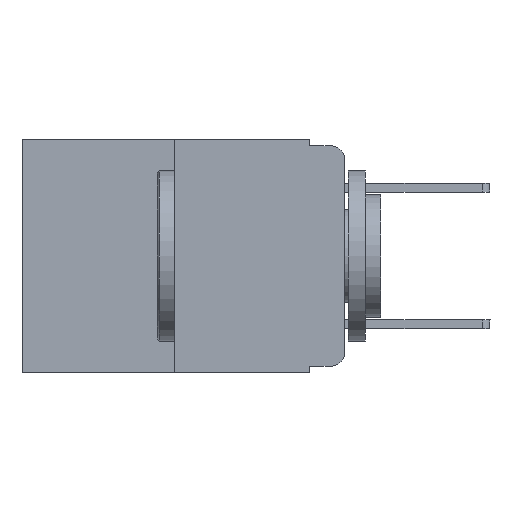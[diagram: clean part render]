
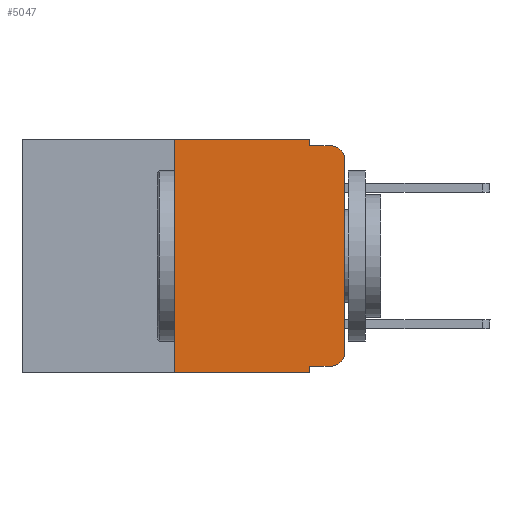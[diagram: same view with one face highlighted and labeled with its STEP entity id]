
A CAD part, left-side view. The second image highlights one B-rep face of the part: STEP entity #5047.
In plain terms, the highlighted planar face has unit normal (-1, 0, 0).
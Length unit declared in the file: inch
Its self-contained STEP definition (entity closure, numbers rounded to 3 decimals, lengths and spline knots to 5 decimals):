
#68 = EDGE_CURVE ( 'NONE', #5482, #10175, #2040, .T. ) ;
#242 = VECTOR ( 'NONE', #7209, 39.37008 ) ;
#312 = DIRECTION ( 'NONE',  ( 0., 0., -1. ) ) ;
#369 = LINE ( 'NONE', #2445, #910 ) ;
#607 = VERTEX_POINT ( 'NONE', #10407 ) ;
#863 = LINE ( 'NONE', #7872, #934 ) ;
#910 = VECTOR ( 'NONE', #6473, 39.37008 ) ;
#934 = VECTOR ( 'NONE', #11919, 39.37008 ) ;
#961 = CARTESIAN_POINT ( 'NONE',  ( 0., 0.25, -0.343 ) ) ;
#1066 = AXIS2_PLACEMENT_3D ( 'NONE', #4052, #8057, #12096 ) ;
#1186 = EDGE_CURVE ( 'NONE', #3997, #4994, #5885, .T. ) ;
#1191 = CARTESIAN_POINT ( 'NONE',  ( 0., 0.25, 0. ) ) ;
#1307 = LINE ( 'NONE', #9463, #3314 ) ;
#1376 = ORIENTED_EDGE ( 'NONE', *, *, #6485, .F. ) ;
#1532 = CIRCLE ( 'NONE', #11672, 0.02 ) ;
#1916 = CARTESIAN_POINT ( 'NONE',  ( 0., 0.051, -0.01 ) ) ;
#1965 = EDGE_CURVE ( 'NONE', #12081, #3352, #12812, .T. ) ;
#2029 = ORIENTED_EDGE ( 'NONE', *, *, #1965, .T. ) ;
#2040 = LINE ( 'NONE', #6078, #9671 ) ;
#2045 = VECTOR ( 'NONE', #3907, 39.37008 ) ;
#2171 = ORIENTED_EDGE ( 'NONE', *, *, #1186, .F. ) ;
#2445 = CARTESIAN_POINT ( 'NONE',  ( 0., 0.473, -0.343 ) ) ;
#2802 = AXIS2_PLACEMENT_3D ( 'NONE', #12356, #10315, #10445 ) ;
#3261 = DIRECTION ( 'NONE',  ( -1., 0., 0. ) ) ;
#3314 = VECTOR ( 'NONE', #312, 39.37008 ) ;
#3338 = ORIENTED_EDGE ( 'NONE', *, *, #6089, .T. ) ;
#3352 = VERTEX_POINT ( 'NONE', #9070 ) ;
#3400 = EDGE_CURVE ( 'NONE', #12081, #607, #1307, .T. ) ;
#3647 = VERTEX_POINT ( 'NONE', #11773 ) ;
#3749 = VERTEX_POINT ( 'NONE', #6932 ) ;
#3871 = DIRECTION ( 'NONE',  ( 0., -1., 0. ) ) ;
#3907 = DIRECTION ( 'NONE',  ( 0., 0., -1. ) ) ;
#3961 = CARTESIAN_POINT ( 'NONE',  ( 0., 0.051, -0.01 ) ) ;
#3977 = CARTESIAN_POINT ( 'NONE',  ( 0., 0.051, 0. ) ) ;
#3997 = VERTEX_POINT ( 'NONE', #8583 ) ;
#4052 = CARTESIAN_POINT ( 'NONE',  ( 0., 0.473, 0. ) ) ;
#4085 = CARTESIAN_POINT ( 'NONE',  ( 0., 0., -0.03 ) ) ;
#4983 = VECTOR ( 'NONE', #3871, 39.37008 ) ;
#4994 = VERTEX_POINT ( 'NONE', #1916 ) ;
#5047 = ADVANCED_FACE ( 'NONE', ( #13112 ), #10133, .F. ) ;
#5181 = EDGE_CURVE ( 'NONE', #3352, #3647, #6169, .T. ) ;
#5482 = VERTEX_POINT ( 'NONE', #961 ) ;
#5505 = ORIENTED_EDGE ( 'NONE', *, *, #11241, .F. ) ;
#5723 = CARTESIAN_POINT ( 'NONE',  ( 0., 0.051, -0.333 ) ) ;
#5885 = LINE ( 'NONE', #3977, #2045 ) ;
#5950 = CARTESIAN_POINT ( 'NONE',  ( 0., 0.051, -0.333 ) ) ;
#6078 = CARTESIAN_POINT ( 'NONE',  ( 0., 0.25, 0. ) ) ;
#6089 = EDGE_CURVE ( 'NONE', #8252, #3749, #1532, .T. ) ;
#6169 = CIRCLE ( 'NONE', #2802, 0.02 ) ;
#6249 = VECTOR ( 'NONE', #8219, 39.37008 ) ;
#6473 = DIRECTION ( 'NONE',  ( 0., -1., 0. ) ) ;
#6485 = EDGE_CURVE ( 'NONE', #10175, #3997, #12310, .T. ) ;
#6719 = ORIENTED_EDGE ( 'NONE', *, *, #3400, .F. ) ;
#6932 = CARTESIAN_POINT ( 'NONE',  ( 0., 0.02, -0.01 ) ) ;
#7209 = DIRECTION ( 'NONE',  ( 0., -1., 0. ) ) ;
#7420 = EDGE_CURVE ( 'NONE', #5482, #607, #369, .T. ) ;
#7872 = CARTESIAN_POINT ( 'NONE',  ( 0., 0., 0. ) ) ;
#7975 = ORIENTED_EDGE ( 'NONE', *, *, #7420, .T. ) ;
#8057 = DIRECTION ( 'NONE',  ( 1., 0., 0. ) ) ;
#8199 = CARTESIAN_POINT ( 'NONE',  ( 0., 0.473, 0. ) ) ;
#8219 = DIRECTION ( 'NONE',  ( 0., -1., 0. ) ) ;
#8252 = VERTEX_POINT ( 'NONE', #4085 ) ;
#8583 = CARTESIAN_POINT ( 'NONE',  ( 0., 0.051, 0. ) ) ;
#8861 = ORIENTED_EDGE ( 'NONE', *, *, #5181, .T. ) ;
#8914 = EDGE_LOOP ( 'NONE', ( #11344, #3338, #5505, #2171, #1376, #10140, #7975, #6719, #2029, #8861 ) ) ;
#9070 = CARTESIAN_POINT ( 'NONE',  ( 0., 0.02, -0.333 ) ) ;
#9216 = LINE ( 'NONE', #3961, #6249 ) ;
#9463 = CARTESIAN_POINT ( 'NONE',  ( 0., 0.051, 0. ) ) ;
#9671 = VECTOR ( 'NONE', #10118, 39.37008 ) ;
#10009 = EDGE_CURVE ( 'NONE', #3647, #8252, #863, .T. ) ;
#10118 = DIRECTION ( 'NONE',  ( 0., 0., 1. ) ) ;
#10133 = PLANE ( 'NONE',  #1066 ) ;
#10140 = ORIENTED_EDGE ( 'NONE', *, *, #68, .F. ) ;
#10175 = VERTEX_POINT ( 'NONE', #1191 ) ;
#10216 = CARTESIAN_POINT ( 'NONE',  ( 0., 0.02, -0.03 ) ) ;
#10315 = DIRECTION ( 'NONE',  ( -1., 0., 0. ) ) ;
#10400 = DIRECTION ( 'NONE',  ( 0., 0., -1. ) ) ;
#10407 = CARTESIAN_POINT ( 'NONE',  ( 0., 0.051, -0.343 ) ) ;
#10445 = DIRECTION ( 'NONE',  ( 0., 0., -1. ) ) ;
#11241 = EDGE_CURVE ( 'NONE', #4994, #3749, #9216, .T. ) ;
#11344 = ORIENTED_EDGE ( 'NONE', *, *, #10009, .T. ) ;
#11672 = AXIS2_PLACEMENT_3D ( 'NONE', #10216, #3261, #10400 ) ;
#11773 = CARTESIAN_POINT ( 'NONE',  ( 0., 0., -0.313 ) ) ;
#11919 = DIRECTION ( 'NONE',  ( 0., 0., 1. ) ) ;
#12081 = VERTEX_POINT ( 'NONE', #5950 ) ;
#12096 = DIRECTION ( 'NONE',  ( 0., 0., -1. ) ) ;
#12310 = LINE ( 'NONE', #8199, #242 ) ;
#12356 = CARTESIAN_POINT ( 'NONE',  ( 0., 0.02, -0.313 ) ) ;
#12812 = LINE ( 'NONE', #5723, #4983 ) ;
#13112 = FACE_OUTER_BOUND ( 'NONE', #8914, .T. ) ;
